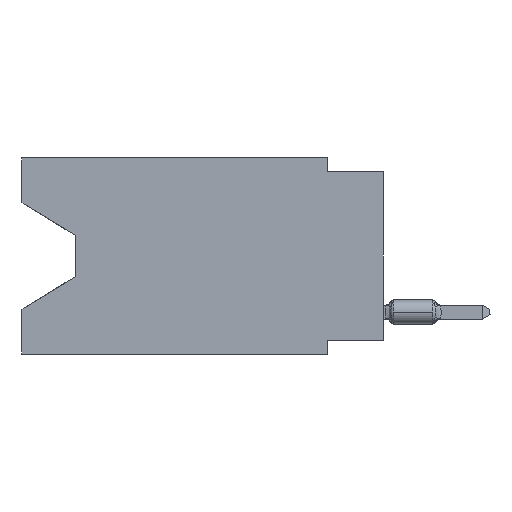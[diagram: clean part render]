
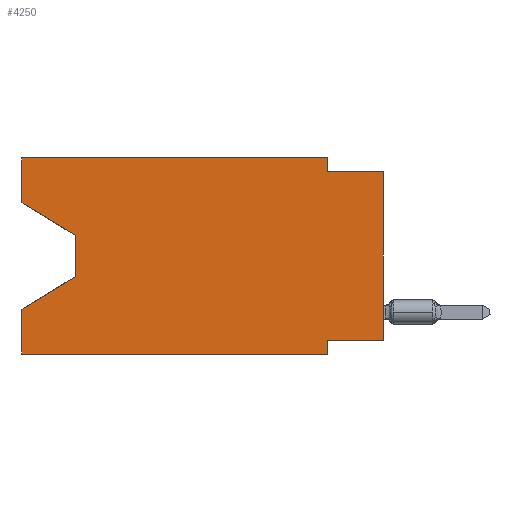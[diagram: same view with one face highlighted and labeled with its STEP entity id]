
A CAD part, left-side view. The second image highlights one B-rep face of the part: STEP entity #4250.
In plain terms, the highlighted planar face has unit normal (-1, 0, 0).
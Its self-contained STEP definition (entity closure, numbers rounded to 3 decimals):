
#992 = DIRECTION ( 'NONE',  ( 0., -0.855, -0.519 ) ) ;
#1332 = LINE ( 'NONE', #46949, #39498 ) ;
#1903 = ORIENTED_EDGE ( 'NONE', *, *, #63545, .F. ) ;
#1972 = DIRECTION ( 'NONE',  ( 0., -1., 0. ) ) ;
#3632 = CARTESIAN_POINT ( 'NONE',  ( 0., 16.383, -8.89 ) ) ;
#3892 = ORIENTED_EDGE ( 'NONE', *, *, #37418, .T. ) ;
#4180 = DIRECTION ( 'NONE',  ( 0., 0., 1. ) ) ;
#4250 = ADVANCED_FACE ( 'NONE', ( #9293 ), #55912, .F. ) ;
#5774 = VERTEX_POINT ( 'NONE', #38807 ) ;
#5957 = CARTESIAN_POINT ( 'NONE',  ( 0., 0., -8.255 ) ) ;
#6667 = VECTOR ( 'NONE', #34082, 1000. ) ;
#7232 = LINE ( 'NONE', #27707, #60489 ) ;
#8960 = DIRECTION ( 'NONE',  ( 1., 0., 0. ) ) ;
#9293 = FACE_OUTER_BOUND ( 'NONE', #62619, .T. ) ;
#9797 = VECTOR ( 'NONE', #42264, 1000. ) ;
#9966 = CARTESIAN_POINT ( 'NONE',  ( 0., 16.383, 0. ) ) ;
#10066 = DIRECTION ( 'NONE',  ( 0., 0., 1. ) ) ;
#12342 = EDGE_CURVE ( 'NONE', #42312, #48036, #42267, .T. ) ;
#12368 = EDGE_CURVE ( 'NONE', #31991, #43509, #62734, .T. ) ;
#12939 = CARTESIAN_POINT ( 'NONE',  ( 0., 16.383, 0. ) ) ;
#12969 = VECTOR ( 'NONE', #41794, 1000. ) ;
#13982 = CARTESIAN_POINT ( 'NONE',  ( 0., 16.383, 0. ) ) ;
#16449 = CARTESIAN_POINT ( 'NONE',  ( 0., 2.54, 0. ) ) ;
#16706 = DIRECTION ( 'NONE',  ( 0., 1., 0. ) ) ;
#16794 = CARTESIAN_POINT ( 'NONE',  ( 0., 16.383, 0. ) ) ;
#17769 = VECTOR ( 'NONE', #10066, 1000. ) ;
#17842 = CARTESIAN_POINT ( 'NONE',  ( 0., 2.54, 0. ) ) ;
#19116 = EDGE_CURVE ( 'NONE', #31991, #5774, #1332, .T. ) ;
#19936 = LINE ( 'NONE', #16449, #9797 ) ;
#20177 = DIRECTION ( 'NONE',  ( 0., 0., -1. ) ) ;
#21360 = LINE ( 'NONE', #27062, #12969 ) ;
#21495 = DIRECTION ( 'NONE',  ( 0., 0., -1. ) ) ;
#22689 = DIRECTION ( 'NONE',  ( 0., -1., 0. ) ) ;
#23115 = VERTEX_POINT ( 'NONE', #28404 ) ;
#24872 = ORIENTED_EDGE ( 'NONE', *, *, #64005, .F. ) ;
#25179 = VERTEX_POINT ( 'NONE', #45116 ) ;
#25809 = EDGE_CURVE ( 'NONE', #25179, #23115, #7232, .T. ) ;
#26850 = CARTESIAN_POINT ( 'NONE',  ( 0., 13.97, -5.385 ) ) ;
#27062 = CARTESIAN_POINT ( 'NONE',  ( 0., 2.54, -8.89 ) ) ;
#27707 = CARTESIAN_POINT ( 'NONE',  ( 0., 0., -0.635 ) ) ;
#28404 = CARTESIAN_POINT ( 'NONE',  ( 0., 0., -0.635 ) ) ;
#29788 = EDGE_CURVE ( 'NONE', #37622, #48036, #40910, .T. ) ;
#30402 = VERTEX_POINT ( 'NONE', #34650 ) ;
#30506 = VECTOR ( 'NONE', #4180, 1000. ) ;
#31991 = VERTEX_POINT ( 'NONE', #49102 ) ;
#32351 = VERTEX_POINT ( 'NONE', #49257 ) ;
#32886 = ORIENTED_EDGE ( 'NONE', *, *, #19116, .T. ) ;
#34082 = DIRECTION ( 'NONE',  ( 0., -1., 0. ) ) ;
#34650 = CARTESIAN_POINT ( 'NONE',  ( 0., 2.54, -8.89 ) ) ;
#36525 = EDGE_CURVE ( 'NONE', #49817, #23115, #55175, .T. ) ;
#36732 = VECTOR ( 'NONE', #57679, 1000. ) ;
#36863 = ORIENTED_EDGE ( 'NONE', *, *, #46465, .F. ) ;
#37418 = EDGE_CURVE ( 'NONE', #37622, #30402, #47931, .T. ) ;
#37622 = VERTEX_POINT ( 'NONE', #3632 ) ;
#38807 = CARTESIAN_POINT ( 'NONE',  ( 0., 13.97, -3.505 ) ) ;
#39498 = VECTOR ( 'NONE', #992, 1000. ) ;
#40910 = LINE ( 'NONE', #41554, #17769 ) ;
#41161 = CARTESIAN_POINT ( 'NONE',  ( 0., 0., -8.255 ) ) ;
#41554 = CARTESIAN_POINT ( 'NONE',  ( 0., 16.383, 0. ) ) ;
#41688 = AXIS2_PLACEMENT_3D ( 'NONE', #9966, #8960, #21495 ) ;
#41794 = DIRECTION ( 'NONE',  ( 0., 0., -1. ) ) ;
#42264 = DIRECTION ( 'NONE',  ( 0., 0., -1. ) ) ;
#42267 = LINE ( 'NONE', #26850, #60334 ) ;
#42312 = VERTEX_POINT ( 'NONE', #53174 ) ;
#42374 = VECTOR ( 'NONE', #1972, 1000. ) ;
#42413 = ORIENTED_EDGE ( 'NONE', *, *, #12368, .F. ) ;
#43015 = VECTOR ( 'NONE', #20177, 1000. ) ;
#43509 = VERTEX_POINT ( 'NONE', #12939 ) ;
#43553 = ORIENTED_EDGE ( 'NONE', *, *, #12342, .T. ) ;
#44538 = CARTESIAN_POINT ( 'NONE',  ( 0., 16.383, -6.852 ) ) ;
#45116 = CARTESIAN_POINT ( 'NONE',  ( 0., 2.54, -0.635 ) ) ;
#45650 = LINE ( 'NONE', #66116, #43015 ) ;
#46332 = ORIENTED_EDGE ( 'NONE', *, *, #65849, .F. ) ;
#46465 = EDGE_CURVE ( 'NONE', #32351, #30402, #21360, .T. ) ;
#46620 = CARTESIAN_POINT ( 'NONE',  ( 0., 16.383, -8.89 ) ) ;
#46949 = CARTESIAN_POINT ( 'NONE',  ( 0., 16.383, -2.038 ) ) ;
#47285 = DIRECTION ( 'NONE',  ( 0., 0.855, -0.519 ) ) ;
#47931 = LINE ( 'NONE', #46620, #42374 ) ;
#48036 = VERTEX_POINT ( 'NONE', #44538 ) ;
#48600 = ORIENTED_EDGE ( 'NONE', *, *, #25809, .F. ) ;
#49102 = CARTESIAN_POINT ( 'NONE',  ( 0., 16.383, -2.038 ) ) ;
#49257 = CARTESIAN_POINT ( 'NONE',  ( 0., 2.54, -8.255 ) ) ;
#49303 = ORIENTED_EDGE ( 'NONE', *, *, #36525, .T. ) ;
#49817 = VERTEX_POINT ( 'NONE', #41161 ) ;
#50805 = CARTESIAN_POINT ( 'NONE',  ( 0., 0., 0. ) ) ;
#51914 = LINE ( 'NONE', #5957, #54848 ) ;
#53174 = CARTESIAN_POINT ( 'NONE',  ( 0., 13.97, -5.385 ) ) ;
#54590 = ORIENTED_EDGE ( 'NONE', *, *, #65590, .T. ) ;
#54848 = VECTOR ( 'NONE', #16706, 1000. ) ;
#55175 = LINE ( 'NONE', #50805, #30506 ) ;
#55912 = PLANE ( 'NONE',  #41688 ) ;
#57679 = DIRECTION ( 'NONE',  ( 0., 0., 1. ) ) ;
#59588 = LINE ( 'NONE', #13982, #6667 ) ;
#59948 = ORIENTED_EDGE ( 'NONE', *, *, #29788, .F. ) ;
#60334 = VECTOR ( 'NONE', #47285, 1000. ) ;
#60489 = VECTOR ( 'NONE', #22689, 1000. ) ;
#62094 = VERTEX_POINT ( 'NONE', #17842 ) ;
#62619 = EDGE_LOOP ( 'NONE', ( #32886, #54590, #43553, #59948, #3892, #36863, #24872, #49303, #48600, #1903, #46332, #42413 ) ) ;
#62734 = LINE ( 'NONE', #16794, #36732 ) ;
#63545 = EDGE_CURVE ( 'NONE', #62094, #25179, #19936, .T. ) ;
#64005 = EDGE_CURVE ( 'NONE', #49817, #32351, #51914, .T. ) ;
#65590 = EDGE_CURVE ( 'NONE', #5774, #42312, #45650, .T. ) ;
#65849 = EDGE_CURVE ( 'NONE', #43509, #62094, #59588, .T. ) ;
#66116 = CARTESIAN_POINT ( 'NONE',  ( 0., 13.97, -3.505 ) ) ;
